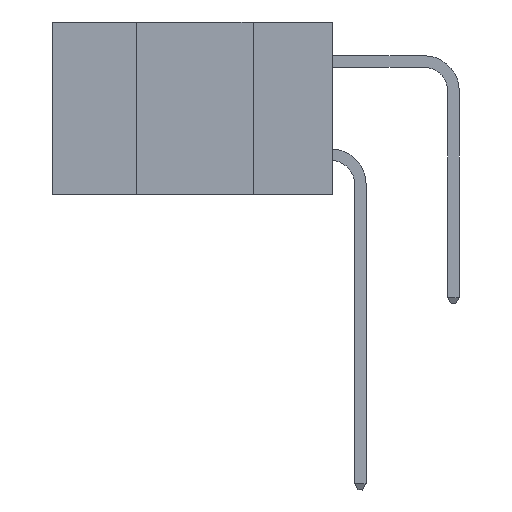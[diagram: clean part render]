
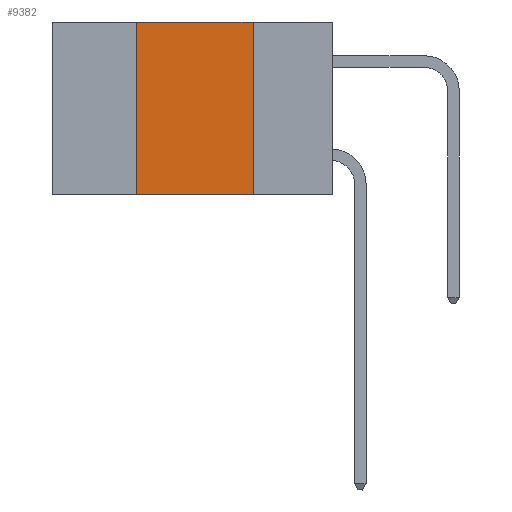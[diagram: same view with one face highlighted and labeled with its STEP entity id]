
A CAD part, left-side view. The second image highlights one B-rep face of the part: STEP entity #9382.
In plain terms, the highlighted planar face has unit normal (-1, 0, 0).
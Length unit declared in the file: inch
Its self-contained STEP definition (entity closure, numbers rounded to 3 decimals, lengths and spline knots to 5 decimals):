
#1009 = ORIENTED_EDGE ( 'NONE', *, *, #14743, .F. ) ;
#1114 = EDGE_CURVE ( 'NONE', #17376, #8160, #16060, .T. ) ;
#1739 = VECTOR ( 'NONE', #3259, 39.37008 ) ;
#2391 = CARTESIAN_POINT ( 'NONE',  ( 0., 0.6, -0.37 ) ) ;
#2916 = PLANE ( 'NONE',  #10985 ) ;
#3259 = DIRECTION ( 'NONE',  ( 0., -1., 0. ) ) ;
#4288 = ORIENTED_EDGE ( 'NONE', *, *, #1114, .T. ) ;
#8160 = VERTEX_POINT ( 'NONE', #15559 ) ;
#8804 = CARTESIAN_POINT ( 'NONE',  ( 0., 0.17, 0. ) ) ;
#9234 = LINE ( 'NONE', #10612, #13061 ) ;
#9382 = ADVANCED_FACE ( 'NONE', ( #10005 ), #2916, .F. ) ;
#9962 = VERTEX_POINT ( 'NONE', #8804 ) ;
#10005 = FACE_OUTER_BOUND ( 'NONE', #15352, .T. ) ;
#10612 = CARTESIAN_POINT ( 'NONE',  ( 0., 0.42, -0.37 ) ) ;
#10985 = AXIS2_PLACEMENT_3D ( 'NONE', #16848, #14334, #17030 ) ;
#11567 = VECTOR ( 'NONE', #13147, 39.37008 ) ;
#11716 = DIRECTION ( 'NONE',  ( 0., 0., 1. ) ) ;
#11952 = CARTESIAN_POINT ( 'NONE',  ( 0., 0.42, 0. ) ) ;
#12227 = VECTOR ( 'NONE', #16682, 39.37008 ) ;
#12272 = EDGE_CURVE ( 'NONE', #17376, #13680, #9234, .T. ) ;
#12628 = CARTESIAN_POINT ( 'NONE',  ( 0., 0.42, -0.37 ) ) ;
#13061 = VECTOR ( 'NONE', #11716, 39.37008 ) ;
#13147 = DIRECTION ( 'NONE',  ( 0., -1., 0. ) ) ;
#13278 = CARTESIAN_POINT ( 'NONE',  ( 0., 0.6, 0. ) ) ;
#13680 = VERTEX_POINT ( 'NONE', #11952 ) ;
#14334 = DIRECTION ( 'NONE',  ( 1., 0., 0. ) ) ;
#14743 = EDGE_CURVE ( 'NONE', #9962, #8160, #15278, .T. ) ;
#15168 = ORIENTED_EDGE ( 'NONE', *, *, #12272, .F. ) ;
#15278 = LINE ( 'NONE', #16592, #12227 ) ;
#15293 = ORIENTED_EDGE ( 'NONE', *, *, #15427, .F. ) ;
#15352 = EDGE_LOOP ( 'NONE', ( #1009, #15293, #15168, #4288 ) ) ;
#15427 = EDGE_CURVE ( 'NONE', #13680, #9962, #15910, .T. ) ;
#15559 = CARTESIAN_POINT ( 'NONE',  ( 0., 0.17, -0.37 ) ) ;
#15910 = LINE ( 'NONE', #13278, #1739 ) ;
#16060 = LINE ( 'NONE', #2391, #11567 ) ;
#16592 = CARTESIAN_POINT ( 'NONE',  ( 0., 0.17, -0.37 ) ) ;
#16682 = DIRECTION ( 'NONE',  ( 0., 0., -1. ) ) ;
#16848 = CARTESIAN_POINT ( 'NONE',  ( 0., 0.6, 0. ) ) ;
#17030 = DIRECTION ( 'NONE',  ( 0., 0., -1. ) ) ;
#17376 = VERTEX_POINT ( 'NONE', #12628 ) ;
